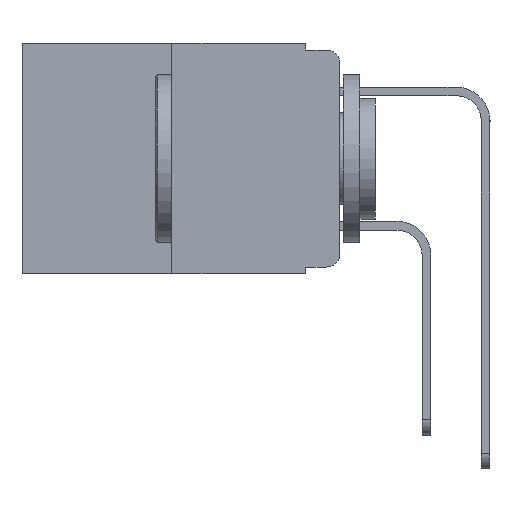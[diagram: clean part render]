
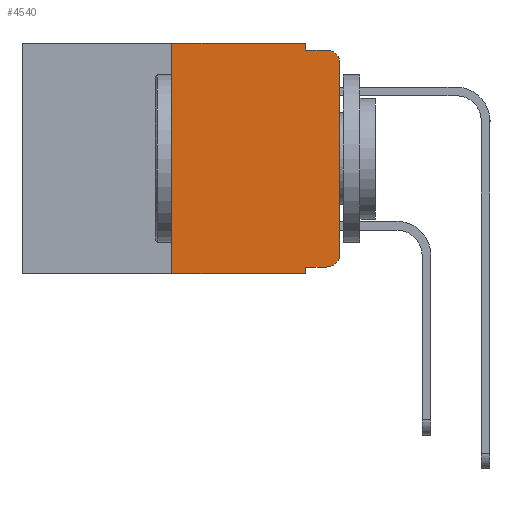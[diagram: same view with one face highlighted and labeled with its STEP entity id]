
A CAD part, left-side view. The second image highlights one B-rep face of the part: STEP entity #4540.
In plain terms, the highlighted planar face has unit normal (-1, 0, 0).
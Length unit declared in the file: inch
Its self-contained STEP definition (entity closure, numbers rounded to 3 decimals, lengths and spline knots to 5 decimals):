
#239 = LINE ( 'NONE', #1123, #11846 ) ;
#312 = CARTESIAN_POINT ( 'NONE',  ( 0., 0.02, -0.03 ) ) ;
#440 = VECTOR ( 'NONE', #8470, 39.37008 ) ;
#592 = CARTESIAN_POINT ( 'NONE',  ( 0., 0., 0. ) ) ;
#612 = EDGE_CURVE ( 'NONE', #8855, #1620, #10739, .T. ) ;
#624 = CARTESIAN_POINT ( 'NONE',  ( 0., 0.25, -0.343 ) ) ;
#801 = ORIENTED_EDGE ( 'NONE', *, *, #5096, .T. ) ;
#905 = EDGE_CURVE ( 'NONE', #2721, #8855, #7268, .T. ) ;
#1123 = CARTESIAN_POINT ( 'NONE',  ( 0., 0.051, -0.333 ) ) ;
#1338 = ORIENTED_EDGE ( 'NONE', *, *, #8709, .T. ) ;
#1491 = VECTOR ( 'NONE', #5672, 39.37008 ) ;
#1501 = CIRCLE ( 'NONE', #2366, 0.02 ) ;
#1576 = DIRECTION ( 'NONE',  ( 0., 0., -1. ) ) ;
#1577 = CARTESIAN_POINT ( 'NONE',  ( 0., 0., -0.03 ) ) ;
#1620 = VERTEX_POINT ( 'NONE', #4566 ) ;
#2366 = AXIS2_PLACEMENT_3D ( 'NONE', #12592, #6065, #13645 ) ;
#2414 = EDGE_LOOP ( 'NONE', ( #8536, #8943, #5124, #11518, #13280, #2700, #2748, #3751, #1338, #801 ) ) ;
#2515 = CARTESIAN_POINT ( 'NONE',  ( 0., 0.473, 0. ) ) ;
#2700 = ORIENTED_EDGE ( 'NONE', *, *, #905, .F. ) ;
#2721 = VERTEX_POINT ( 'NONE', #624 ) ;
#2748 = ORIENTED_EDGE ( 'NONE', *, *, #11672, .T. ) ;
#2862 = VERTEX_POINT ( 'NONE', #4412 ) ;
#3262 = DIRECTION ( 'NONE',  ( 0., -1., 0. ) ) ;
#3527 = CARTESIAN_POINT ( 'NONE',  ( 0., 0.02, -0.01 ) ) ;
#3663 = LINE ( 'NONE', #592, #440 ) ;
#3751 = ORIENTED_EDGE ( 'NONE', *, *, #10924, .F. ) ;
#3894 = CARTESIAN_POINT ( 'NONE',  ( 0., 0.02, -0.333 ) ) ;
#4085 = PLANE ( 'NONE',  #8035 ) ;
#4097 = EDGE_CURVE ( 'NONE', #1620, #4107, #8493, .T. ) ;
#4107 = VERTEX_POINT ( 'NONE', #12038 ) ;
#4160 = DIRECTION ( 'NONE',  ( 0., 0., -1. ) ) ;
#4412 = CARTESIAN_POINT ( 'NONE',  ( 0., 0.051, -0.343 ) ) ;
#4437 = VECTOR ( 'NONE', #8513, 39.37008 ) ;
#4540 = ADVANCED_FACE ( 'NONE', ( #8831 ), #4085, .F. ) ;
#4566 = CARTESIAN_POINT ( 'NONE',  ( 0., 0.051, 0. ) ) ;
#4652 = VECTOR ( 'NONE', #3262, 39.37008 ) ;
#4959 = VECTOR ( 'NONE', #11594, 39.37008 ) ;
#5096 = EDGE_CURVE ( 'NONE', #7614, #9387, #1501, .T. ) ;
#5124 = ORIENTED_EDGE ( 'NONE', *, *, #5535, .F. ) ;
#5178 = VECTOR ( 'NONE', #4160, 39.37008 ) ;
#5179 = DIRECTION ( 'NONE',  ( 0., 0., -1. ) ) ;
#5535 = EDGE_CURVE ( 'NONE', #4107, #8031, #10369, .T. ) ;
#5672 = DIRECTION ( 'NONE',  ( 0., -1., 0. ) ) ;
#5814 = CARTESIAN_POINT ( 'NONE',  ( 0., 0.051, -0.333 ) ) ;
#6065 = DIRECTION ( 'NONE',  ( -1., 0., 0. ) ) ;
#6974 = EDGE_CURVE ( 'NONE', #11437, #8031, #7224, .T. ) ;
#7224 = CIRCLE ( 'NONE', #8808, 0.02 ) ;
#7268 = LINE ( 'NONE', #8292, #4437 ) ;
#7614 = VERTEX_POINT ( 'NONE', #3894 ) ;
#8031 = VERTEX_POINT ( 'NONE', #3527 ) ;
#8035 = AXIS2_PLACEMENT_3D ( 'NONE', #10600, #11706, #5179 ) ;
#8066 = CARTESIAN_POINT ( 'NONE',  ( 0., 0.25, 0. ) ) ;
#8224 = DIRECTION ( 'NONE',  ( -1., 0., 0. ) ) ;
#8292 = CARTESIAN_POINT ( 'NONE',  ( 0., 0.25, 0. ) ) ;
#8422 = EDGE_CURVE ( 'NONE', #9387, #11437, #3663, .T. ) ;
#8470 = DIRECTION ( 'NONE',  ( 0., 0., 1. ) ) ;
#8493 = LINE ( 'NONE', #10941, #11434 ) ;
#8513 = DIRECTION ( 'NONE',  ( 0., 0., 1. ) ) ;
#8536 = ORIENTED_EDGE ( 'NONE', *, *, #8422, .T. ) ;
#8709 = EDGE_CURVE ( 'NONE', #9343, #7614, #239, .T. ) ;
#8808 = AXIS2_PLACEMENT_3D ( 'NONE', #312, #8224, #1576 ) ;
#8831 = FACE_OUTER_BOUND ( 'NONE', #2414, .T. ) ;
#8855 = VERTEX_POINT ( 'NONE', #8066 ) ;
#8943 = ORIENTED_EDGE ( 'NONE', *, *, #6974, .T. ) ;
#9343 = VERTEX_POINT ( 'NONE', #5814 ) ;
#9387 = VERTEX_POINT ( 'NONE', #11343 ) ;
#9628 = CARTESIAN_POINT ( 'NONE',  ( 0., 0.051, 0. ) ) ;
#9797 = CARTESIAN_POINT ( 'NONE',  ( 0., 0.473, -0.343 ) ) ;
#10087 = LINE ( 'NONE', #9797, #4652 ) ;
#10369 = LINE ( 'NONE', #12209, #1491 ) ;
#10600 = CARTESIAN_POINT ( 'NONE',  ( 0., 0.473, 0. ) ) ;
#10739 = LINE ( 'NONE', #2515, #4959 ) ;
#10924 = EDGE_CURVE ( 'NONE', #9343, #2862, #10965, .T. ) ;
#10941 = CARTESIAN_POINT ( 'NONE',  ( 0., 0.051, 0. ) ) ;
#10965 = LINE ( 'NONE', #9628, #5178 ) ;
#11343 = CARTESIAN_POINT ( 'NONE',  ( 0., 0., -0.313 ) ) ;
#11434 = VECTOR ( 'NONE', #14054, 39.37008 ) ;
#11437 = VERTEX_POINT ( 'NONE', #1577 ) ;
#11518 = ORIENTED_EDGE ( 'NONE', *, *, #4097, .F. ) ;
#11594 = DIRECTION ( 'NONE',  ( 0., -1., 0. ) ) ;
#11672 = EDGE_CURVE ( 'NONE', #2721, #2862, #10087, .T. ) ;
#11706 = DIRECTION ( 'NONE',  ( 1., 0., 0. ) ) ;
#11846 = VECTOR ( 'NONE', #14321, 39.37008 ) ;
#12038 = CARTESIAN_POINT ( 'NONE',  ( 0., 0.051, -0.01 ) ) ;
#12209 = CARTESIAN_POINT ( 'NONE',  ( 0., 0.051, -0.01 ) ) ;
#12592 = CARTESIAN_POINT ( 'NONE',  ( 0., 0.02, -0.313 ) ) ;
#13280 = ORIENTED_EDGE ( 'NONE', *, *, #612, .F. ) ;
#13645 = DIRECTION ( 'NONE',  ( 0., 0., -1. ) ) ;
#14054 = DIRECTION ( 'NONE',  ( 0., 0., -1. ) ) ;
#14321 = DIRECTION ( 'NONE',  ( 0., -1., 0. ) ) ;
